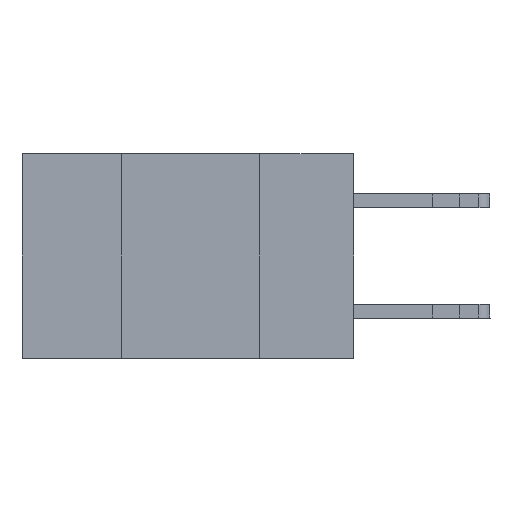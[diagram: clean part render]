
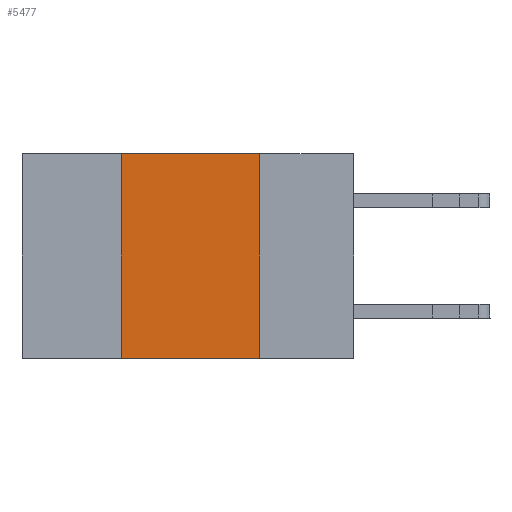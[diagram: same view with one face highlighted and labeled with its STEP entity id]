
A CAD part, left-side view. The second image highlights one B-rep face of the part: STEP entity #5477.
In plain terms, the highlighted planar face has unit normal (-1, 0, 0).
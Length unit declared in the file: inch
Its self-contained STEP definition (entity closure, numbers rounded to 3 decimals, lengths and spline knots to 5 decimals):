
#792 = EDGE_CURVE ( 'NONE', #10145, #2746, #24236, .T. ) ;
#1215 = ORIENTED_EDGE ( 'NONE', *, *, #5225, .F. ) ;
#1625 = VECTOR ( 'NONE', #34026, 39.37008 ) ;
#2746 = VERTEX_POINT ( 'NONE', #25845 ) ;
#4265 = CARTESIAN_POINT ( 'NONE',  ( 0., 0.42, 0. ) ) ;
#5225 = EDGE_CURVE ( 'NONE', #13272, #10145, #18530, .T. ) ;
#5477 = ADVANCED_FACE ( 'NONE', ( #22737 ), #27550, .F. ) ;
#7830 = EDGE_CURVE ( 'NONE', #2746, #23062, #25959, .T. ) ;
#7902 = ORIENTED_EDGE ( 'NONE', *, *, #792, .F. ) ;
#9281 = DIRECTION ( 'NONE',  ( 0., 0., -1. ) ) ;
#9998 = LINE ( 'NONE', #33562, #1625 ) ;
#10145 = VERTEX_POINT ( 'NONE', #4265 ) ;
#10542 = AXIS2_PLACEMENT_3D ( 'NONE', #21959, #30250, #27417 ) ;
#10751 = VECTOR ( 'NONE', #9281, 39.37008 ) ;
#11234 = CARTESIAN_POINT ( 'NONE',  ( 0., 0.42, -0.37 ) ) ;
#11302 = EDGE_CURVE ( 'NONE', #13272, #23062, #9998, .T. ) ;
#13272 = VERTEX_POINT ( 'NONE', #11234 ) ;
#18530 = LINE ( 'NONE', #26553, #26190 ) ;
#20297 = ORIENTED_EDGE ( 'NONE', *, *, #11302, .T. ) ;
#21959 = CARTESIAN_POINT ( 'NONE',  ( 0., 0.6, 0. ) ) ;
#22092 = VECTOR ( 'NONE', #34668, 39.37008 ) ;
#22737 = FACE_OUTER_BOUND ( 'NONE', #29001, .T. ) ;
#23062 = VERTEX_POINT ( 'NONE', #27253 ) ;
#23654 = DIRECTION ( 'NONE',  ( 0., 0., 1. ) ) ;
#24236 = LINE ( 'NONE', #29586, #22092 ) ;
#25845 = CARTESIAN_POINT ( 'NONE',  ( 0., 0.17, 0. ) ) ;
#25959 = LINE ( 'NONE', #33424, #10751 ) ;
#26190 = VECTOR ( 'NONE', #23654, 39.37008 ) ;
#26553 = CARTESIAN_POINT ( 'NONE',  ( 0., 0.42, 0. ) ) ;
#27058 = ORIENTED_EDGE ( 'NONE', *, *, #7830, .F. ) ;
#27253 = CARTESIAN_POINT ( 'NONE',  ( 0., 0.17, -0.37 ) ) ;
#27417 = DIRECTION ( 'NONE',  ( 0., 0., -1. ) ) ;
#27550 = PLANE ( 'NONE',  #10542 ) ;
#29001 = EDGE_LOOP ( 'NONE', ( #27058, #7902, #1215, #20297 ) ) ;
#29586 = CARTESIAN_POINT ( 'NONE',  ( 0., 0.6, 0. ) ) ;
#30250 = DIRECTION ( 'NONE',  ( 1., 0., 0. ) ) ;
#33424 = CARTESIAN_POINT ( 'NONE',  ( 0., 0.17, 0. ) ) ;
#33562 = CARTESIAN_POINT ( 'NONE',  ( 0., 0.6, -0.37 ) ) ;
#34026 = DIRECTION ( 'NONE',  ( 0., -1., 0. ) ) ;
#34668 = DIRECTION ( 'NONE',  ( 0., -1., 0. ) ) ;
